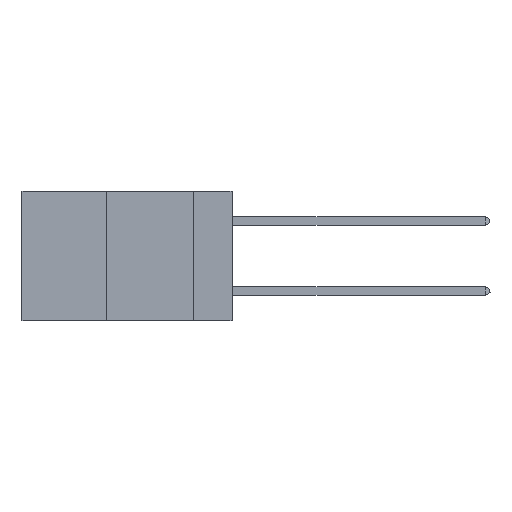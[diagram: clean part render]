
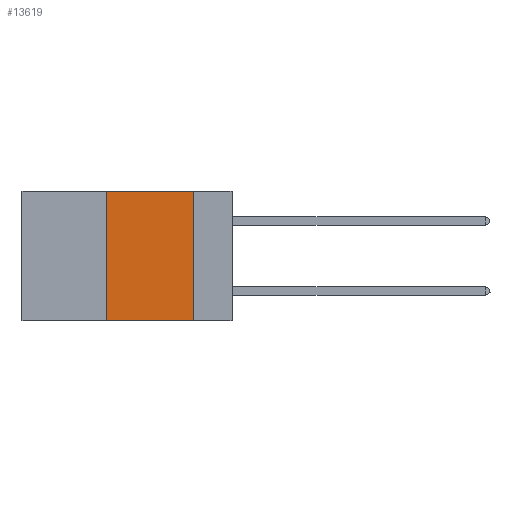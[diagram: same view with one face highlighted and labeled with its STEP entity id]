
A CAD part, left-side view. The second image highlights one B-rep face of the part: STEP entity #13619.
In plain terms, the highlighted planar face has unit normal (-1, 0, 0).
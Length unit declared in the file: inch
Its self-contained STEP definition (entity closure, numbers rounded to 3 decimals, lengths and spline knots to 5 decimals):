
#645 = DIRECTION ( 'NONE',  ( 0., -1., 0. ) ) ;
#1015 = CARTESIAN_POINT ( 'NONE',  ( 0., 0.11, -0.37 ) ) ;
#1123 = VECTOR ( 'NONE', #7634, 39.37008 ) ;
#1457 = VERTEX_POINT ( 'NONE', #6948 ) ;
#1950 = CARTESIAN_POINT ( 'NONE',  ( 0., 0.11, 0. ) ) ;
#2335 = DIRECTION ( 'NONE',  ( 0., -1., 0. ) ) ;
#2901 = DIRECTION ( 'NONE',  ( 1., 0., 0. ) ) ;
#3300 = VECTOR ( 'NONE', #2335, 39.37008 ) ;
#3611 = EDGE_CURVE ( 'NONE', #18564, #19280, #14910, .T. ) ;
#4146 = EDGE_LOOP ( 'NONE', ( #19319, #19332, #18906, #16841 ) ) ;
#4569 = LINE ( 'NONE', #14426, #3300 ) ;
#6274 = VECTOR ( 'NONE', #645, 39.37008 ) ;
#6948 = CARTESIAN_POINT ( 'NONE',  ( 0., 0.36, -0.37 ) ) ;
#7634 = DIRECTION ( 'NONE',  ( 0., 0., -1. ) ) ;
#8598 = CARTESIAN_POINT ( 'NONE',  ( 0., 0.6, 0. ) ) ;
#9199 = DIRECTION ( 'NONE',  ( 0., 0., -1. ) ) ;
#9219 = VERTEX_POINT ( 'NONE', #12639 ) ;
#10391 = EDGE_CURVE ( 'NONE', #1457, #9219, #23661, .T. ) ;
#11228 = PLANE ( 'NONE',  #11996 ) ;
#11996 = AXIS2_PLACEMENT_3D ( 'NONE', #14987, #2901, #9199 ) ;
#12391 = VECTOR ( 'NONE', #15823, 39.37008 ) ;
#12639 = CARTESIAN_POINT ( 'NONE',  ( 0., 0.36, 0. ) ) ;
#13619 = ADVANCED_FACE ( 'NONE', ( #16053 ), #11228, .F. ) ;
#13770 = CARTESIAN_POINT ( 'NONE',  ( 0., 0.11, 0. ) ) ;
#14426 = CARTESIAN_POINT ( 'NONE',  ( 0., 0.6, -0.37 ) ) ;
#14910 = LINE ( 'NONE', #1950, #1123 ) ;
#14987 = CARTESIAN_POINT ( 'NONE',  ( 0., 0.6, 0. ) ) ;
#15823 = DIRECTION ( 'NONE',  ( 0., 0., 1. ) ) ;
#16053 = FACE_OUTER_BOUND ( 'NONE', #4146, .T. ) ;
#16841 = ORIENTED_EDGE ( 'NONE', *, *, #21733, .T. ) ;
#18462 = LINE ( 'NONE', #8598, #6274 ) ;
#18564 = VERTEX_POINT ( 'NONE', #13770 ) ;
#18906 = ORIENTED_EDGE ( 'NONE', *, *, #10391, .F. ) ;
#19280 = VERTEX_POINT ( 'NONE', #1015 ) ;
#19319 = ORIENTED_EDGE ( 'NONE', *, *, #3611, .F. ) ;
#19332 = ORIENTED_EDGE ( 'NONE', *, *, #20030, .F. ) ;
#20030 = EDGE_CURVE ( 'NONE', #9219, #18564, #18462, .T. ) ;
#21733 = EDGE_CURVE ( 'NONE', #1457, #19280, #4569, .T. ) ;
#23661 = LINE ( 'NONE', #25521, #12391 ) ;
#25521 = CARTESIAN_POINT ( 'NONE',  ( 0., 0.36, 0. ) ) ;
